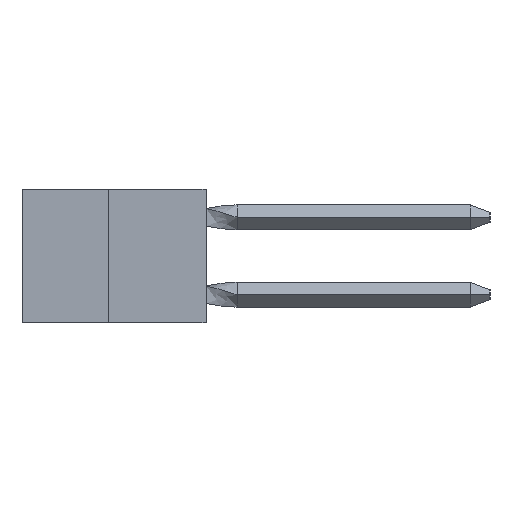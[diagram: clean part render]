
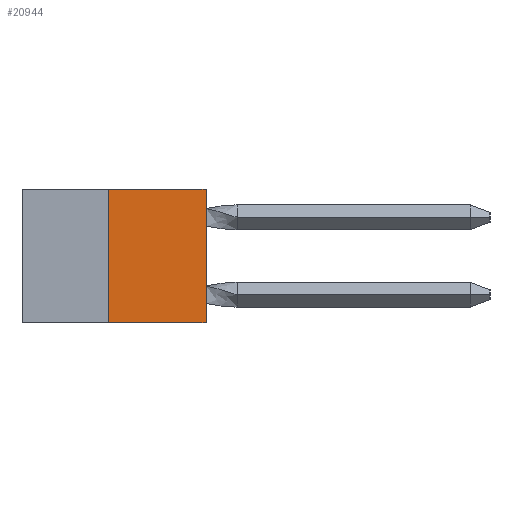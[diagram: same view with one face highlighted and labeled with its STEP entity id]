
A CAD part, left-side view. The second image highlights one B-rep face of the part: STEP entity #20944.
In plain terms, the highlighted planar face has unit normal (-1, 0, 0).
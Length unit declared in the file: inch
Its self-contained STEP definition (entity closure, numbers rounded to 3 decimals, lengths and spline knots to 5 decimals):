
#140 = VECTOR ( 'NONE', #4544, 39.37008 ) ;
#263 = EDGE_CURVE ( 'NONE', #6633, #1274, #6455, .T. ) ;
#1041 = EDGE_CURVE ( 'NONE', #1274, #11871, #23995, .T. ) ;
#1274 = VERTEX_POINT ( 'NONE', #23821 ) ;
#3144 = DIRECTION ( 'NONE',  ( 0., -1., 0. ) ) ;
#4068 = FACE_OUTER_BOUND ( 'NONE', #9531, .T. ) ;
#4544 = DIRECTION ( 'NONE',  ( 0., -1., 0. ) ) ;
#4641 = AXIS2_PLACEMENT_3D ( 'NONE', #5403, #7212, #24030 ) ;
#5403 = CARTESIAN_POINT ( 'NONE',  ( 0., 0.473, 0. ) ) ;
#6455 = LINE ( 'NONE', #16962, #22173 ) ;
#6633 = VERTEX_POINT ( 'NONE', #19511 ) ;
#7212 = DIRECTION ( 'NONE',  ( 1., 0., 0. ) ) ;
#7262 = VERTEX_POINT ( 'NONE', #16074 ) ;
#9531 = EDGE_LOOP ( 'NONE', ( #9579, #18801, #16437, #23289 ) ) ;
#9537 = CARTESIAN_POINT ( 'NONE',  ( 0., 0., 0. ) ) ;
#9579 = ORIENTED_EDGE ( 'NONE', *, *, #1041, .F. ) ;
#11864 = CARTESIAN_POINT ( 'NONE',  ( 0., 0.473, 0. ) ) ;
#11871 = VERTEX_POINT ( 'NONE', #9537 ) ;
#13676 = VECTOR ( 'NONE', #3144, 39.37008 ) ;
#14296 = CARTESIAN_POINT ( 'NONE',  ( 0., 0.473, -0.343 ) ) ;
#15536 = LINE ( 'NONE', #17840, #18735 ) ;
#16074 = CARTESIAN_POINT ( 'NONE',  ( 0., 0., -0.343 ) ) ;
#16437 = ORIENTED_EDGE ( 'NONE', *, *, #20888, .T. ) ;
#16962 = CARTESIAN_POINT ( 'NONE',  ( 0., 0.25, 0. ) ) ;
#17840 = CARTESIAN_POINT ( 'NONE',  ( 0., 0., 0. ) ) ;
#18735 = VECTOR ( 'NONE', #21713, 39.37008 ) ;
#18801 = ORIENTED_EDGE ( 'NONE', *, *, #263, .F. ) ;
#18901 = DIRECTION ( 'NONE',  ( 0., 0., 1. ) ) ;
#19285 = EDGE_CURVE ( 'NONE', #7262, #11871, #15536, .T. ) ;
#19511 = CARTESIAN_POINT ( 'NONE',  ( 0., 0.25, -0.343 ) ) ;
#20888 = EDGE_CURVE ( 'NONE', #6633, #7262, #23871, .T. ) ;
#20944 = ADVANCED_FACE ( 'NONE', ( #4068 ), #22104, .F. ) ;
#21713 = DIRECTION ( 'NONE',  ( 0., 0., 1. ) ) ;
#22104 = PLANE ( 'NONE',  #4641 ) ;
#22173 = VECTOR ( 'NONE', #18901, 39.37008 ) ;
#23289 = ORIENTED_EDGE ( 'NONE', *, *, #19285, .T. ) ;
#23821 = CARTESIAN_POINT ( 'NONE',  ( 0., 0.25, 0. ) ) ;
#23871 = LINE ( 'NONE', #14296, #13676 ) ;
#23995 = LINE ( 'NONE', #11864, #140 ) ;
#24030 = DIRECTION ( 'NONE',  ( 0., 0., -1. ) ) ;
